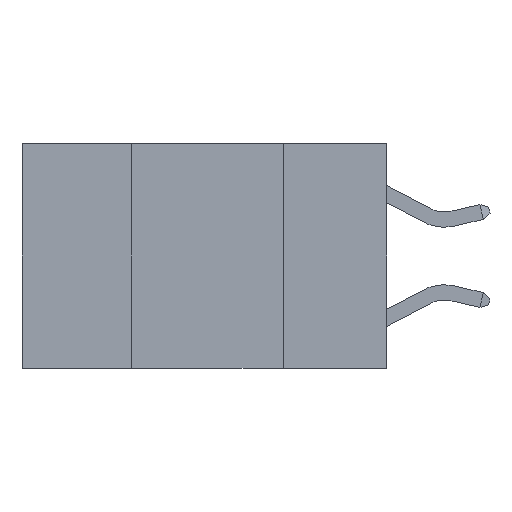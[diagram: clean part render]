
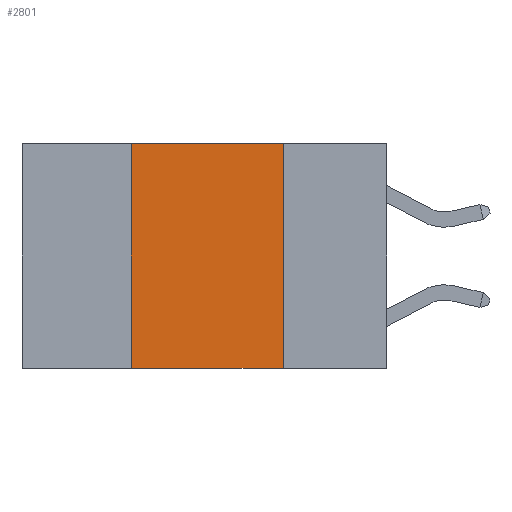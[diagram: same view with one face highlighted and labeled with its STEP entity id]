
A CAD part, left-side view. The second image highlights one B-rep face of the part: STEP entity #2801.
In plain terms, the highlighted planar face has unit normal (-1, 0, 0).
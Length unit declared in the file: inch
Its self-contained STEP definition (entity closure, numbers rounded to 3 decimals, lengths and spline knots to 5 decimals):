
#73 = LINE ( 'NONE', #8117, #2249 ) ;
#584 = PLANE ( 'NONE',  #9539 ) ;
#740 = VERTEX_POINT ( 'NONE', #1076 ) ;
#1076 = CARTESIAN_POINT ( 'NONE',  ( 0., 0.17, 0. ) ) ;
#1547 = DIRECTION ( 'NONE',  ( 1., 0., 0. ) ) ;
#1577 = CARTESIAN_POINT ( 'NONE',  ( 0., 0.17, 0. ) ) ;
#1616 = ORIENTED_EDGE ( 'NONE', *, *, #5048, .F. ) ;
#1716 = CARTESIAN_POINT ( 'NONE',  ( 0., 0.6, 0. ) ) ;
#1905 = ORIENTED_EDGE ( 'NONE', *, *, #5070, .T. ) ;
#2249 = VECTOR ( 'NONE', #2508, 39.37008 ) ;
#2508 = DIRECTION ( 'NONE',  ( 0., -1., 0. ) ) ;
#2510 = VECTOR ( 'NONE', #4977, 39.37008 ) ;
#2801 = ADVANCED_FACE ( 'NONE', ( #7140 ), #584, .F. ) ;
#3456 = LINE ( 'NONE', #1716, #9583 ) ;
#3843 = CARTESIAN_POINT ( 'NONE',  ( 0., 0.17, -0.37 ) ) ;
#3899 = ORIENTED_EDGE ( 'NONE', *, *, #3978, .F. ) ;
#3978 = EDGE_CURVE ( 'NONE', #7286, #740, #3456, .T. ) ;
#4861 = VERTEX_POINT ( 'NONE', #3843 ) ;
#4977 = DIRECTION ( 'NONE',  ( 0., 0., 1. ) ) ;
#4981 = LINE ( 'NONE', #1577, #6814 ) ;
#5048 = EDGE_CURVE ( 'NONE', #740, #4861, #4981, .T. ) ;
#5066 = EDGE_CURVE ( 'NONE', #8869, #7286, #8941, .T. ) ;
#5070 = EDGE_CURVE ( 'NONE', #8869, #4861, #73, .T. ) ;
#5641 = EDGE_LOOP ( 'NONE', ( #1616, #3899, #10239, #1905 ) ) ;
#5754 = DIRECTION ( 'NONE',  ( 0., 0., -1. ) ) ;
#6502 = CARTESIAN_POINT ( 'NONE',  ( 0., 0.6, 0. ) ) ;
#6814 = VECTOR ( 'NONE', #5754, 39.37008 ) ;
#6827 = CARTESIAN_POINT ( 'NONE',  ( 0., 0.42, 0. ) ) ;
#7140 = FACE_OUTER_BOUND ( 'NONE', #5641, .T. ) ;
#7273 = DIRECTION ( 'NONE',  ( 0., 0., -1. ) ) ;
#7286 = VERTEX_POINT ( 'NONE', #6827 ) ;
#8117 = CARTESIAN_POINT ( 'NONE',  ( 0., 0.6, -0.37 ) ) ;
#8242 = DIRECTION ( 'NONE',  ( 0., -1., 0. ) ) ;
#8869 = VERTEX_POINT ( 'NONE', #9378 ) ;
#8941 = LINE ( 'NONE', #10476, #2510 ) ;
#9378 = CARTESIAN_POINT ( 'NONE',  ( 0., 0.42, -0.37 ) ) ;
#9539 = AXIS2_PLACEMENT_3D ( 'NONE', #6502, #1547, #7273 ) ;
#9583 = VECTOR ( 'NONE', #8242, 39.37008 ) ;
#10239 = ORIENTED_EDGE ( 'NONE', *, *, #5066, .F. ) ;
#10476 = CARTESIAN_POINT ( 'NONE',  ( 0., 0.42, 0. ) ) ;
